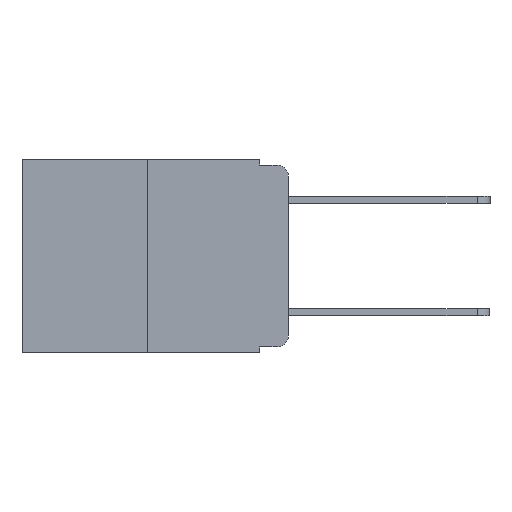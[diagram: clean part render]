
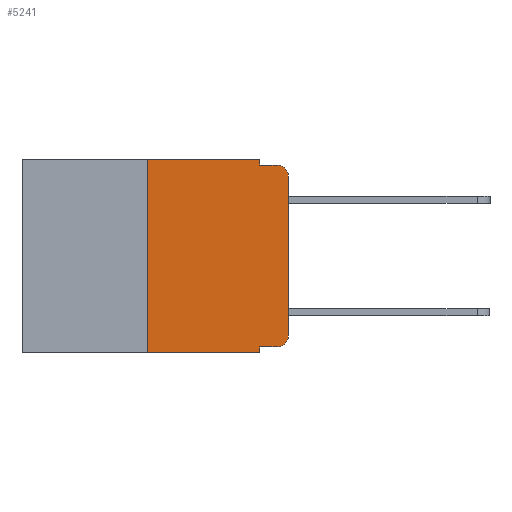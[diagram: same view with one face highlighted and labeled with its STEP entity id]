
A CAD part, left-side view. The second image highlights one B-rep face of the part: STEP entity #5241.
In plain terms, the highlighted planar face has unit normal (-1, 0, 0).
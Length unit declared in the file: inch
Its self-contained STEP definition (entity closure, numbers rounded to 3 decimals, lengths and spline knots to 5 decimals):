
#157 = ORIENTED_EDGE ( 'NONE', *, *, #12236, .F. ) ;
#330 = EDGE_CURVE ( 'NONE', #16093, #11026, #552, .T. ) ;
#552 = LINE ( 'NONE', #17860, #9803 ) ;
#827 = AXIS2_PLACEMENT_3D ( 'NONE', #8892, #20573, #10691 ) ;
#1043 = VERTEX_POINT ( 'NONE', #3173 ) ;
#1145 = VERTEX_POINT ( 'NONE', #20586 ) ;
#1331 = EDGE_CURVE ( 'NONE', #15714, #16093, #13649, .T. ) ;
#1459 = LINE ( 'NONE', #8725, #14645 ) ;
#1630 = CARTESIAN_POINT ( 'NONE',  ( 0., 0.051, -0.333 ) ) ;
#2028 = VECTOR ( 'NONE', #16194, 39.37008 ) ;
#2191 = LINE ( 'NONE', #5204, #19053 ) ;
#2427 = DIRECTION ( 'NONE',  ( 0., 0., 1. ) ) ;
#3173 = CARTESIAN_POINT ( 'NONE',  ( 0., 0., -0.03 ) ) ;
#3844 = LINE ( 'NONE', #4160, #21431 ) ;
#4160 = CARTESIAN_POINT ( 'NONE',  ( 0., 0.25, 0. ) ) ;
#4267 = FACE_OUTER_BOUND ( 'NONE', #19281, .T. ) ;
#4420 = VERTEX_POINT ( 'NONE', #1630 ) ;
#5001 = LINE ( 'NONE', #18997, #13856 ) ;
#5071 = DIRECTION ( 'NONE',  ( 0., 0., -1. ) ) ;
#5204 = CARTESIAN_POINT ( 'NONE',  ( 0., 0.051, -0.333 ) ) ;
#5241 = ADVANCED_FACE ( 'NONE', ( #4267 ), #18147, .F. ) ;
#6113 = ORIENTED_EDGE ( 'NONE', *, *, #330, .F. ) ;
#7399 = DIRECTION ( 'NONE',  ( 0., -1., 0. ) ) ;
#7529 = ORIENTED_EDGE ( 'NONE', *, *, #20690, .T. ) ;
#7534 = CARTESIAN_POINT ( 'NONE',  ( 0., 0.051, -0.01 ) ) ;
#7612 = DIRECTION ( 'NONE',  ( -1., 0., 0. ) ) ;
#8083 = AXIS2_PLACEMENT_3D ( 'NONE', #16545, #19755, #9755 ) ;
#8124 = CARTESIAN_POINT ( 'NONE',  ( 0., 0.051, 0. ) ) ;
#8725 = CARTESIAN_POINT ( 'NONE',  ( 0., 0.051, 0. ) ) ;
#8892 = CARTESIAN_POINT ( 'NONE',  ( 0., 0.02, -0.03 ) ) ;
#8924 = DIRECTION ( 'NONE',  ( 0., -1., 0. ) ) ;
#9149 = EDGE_CURVE ( 'NONE', #18363, #21343, #10734, .T. ) ;
#9168 = CARTESIAN_POINT ( 'NONE',  ( 0., 0.25, 0. ) ) ;
#9550 = CIRCLE ( 'NONE', #12387, 0.02 ) ;
#9646 = ORIENTED_EDGE ( 'NONE', *, *, #16499, .T. ) ;
#9725 = ORIENTED_EDGE ( 'NONE', *, *, #1331, .F. ) ;
#9755 = DIRECTION ( 'NONE',  ( 0., 0., -1. ) ) ;
#9803 = VECTOR ( 'NONE', #7399, 39.37008 ) ;
#10123 = EDGE_CURVE ( 'NONE', #1043, #11026, #12864, .T. ) ;
#10248 = CARTESIAN_POINT ( 'NONE',  ( 0., 0.02, -0.333 ) ) ;
#10691 = DIRECTION ( 'NONE',  ( 0., 0., -1. ) ) ;
#10734 = LINE ( 'NONE', #14883, #19043 ) ;
#11026 = VERTEX_POINT ( 'NONE', #15997 ) ;
#11034 = ORIENTED_EDGE ( 'NONE', *, *, #11558, .F. ) ;
#11558 = EDGE_CURVE ( 'NONE', #4420, #21343, #1459, .T. ) ;
#11722 = VERTEX_POINT ( 'NONE', #9168 ) ;
#12236 = EDGE_CURVE ( 'NONE', #11722, #15714, #5001, .T. ) ;
#12387 = AXIS2_PLACEMENT_3D ( 'NONE', #17790, #7612, #19386 ) ;
#12864 = CIRCLE ( 'NONE', #827, 0.02 ) ;
#13649 = LINE ( 'NONE', #14175, #22176 ) ;
#13788 = CARTESIAN_POINT ( 'NONE',  ( 0., 0.25, -0.343 ) ) ;
#13856 = VECTOR ( 'NONE', #8924, 39.37008 ) ;
#14175 = CARTESIAN_POINT ( 'NONE',  ( 0., 0.051, 0. ) ) ;
#14541 = CARTESIAN_POINT ( 'NONE',  ( 0., 0., 0. ) ) ;
#14645 = VECTOR ( 'NONE', #18827, 39.37008 ) ;
#14883 = CARTESIAN_POINT ( 'NONE',  ( 0., 0.473, -0.343 ) ) ;
#15157 = VERTEX_POINT ( 'NONE', #10248 ) ;
#15586 = ORIENTED_EDGE ( 'NONE', *, *, #17955, .T. ) ;
#15714 = VERTEX_POINT ( 'NONE', #8124 ) ;
#15997 = CARTESIAN_POINT ( 'NONE',  ( 0., 0.02, -0.01 ) ) ;
#16093 = VERTEX_POINT ( 'NONE', #7534 ) ;
#16161 = LINE ( 'NONE', #14541, #2028 ) ;
#16178 = CARTESIAN_POINT ( 'NONE',  ( 0., 0.051, -0.343 ) ) ;
#16194 = DIRECTION ( 'NONE',  ( 0., 0., 1. ) ) ;
#16499 = EDGE_CURVE ( 'NONE', #4420, #15157, #2191, .T. ) ;
#16545 = CARTESIAN_POINT ( 'NONE',  ( 0., 0.473, 0. ) ) ;
#17790 = CARTESIAN_POINT ( 'NONE',  ( 0., 0.02, -0.313 ) ) ;
#17860 = CARTESIAN_POINT ( 'NONE',  ( 0., 0.051, -0.01 ) ) ;
#17955 = EDGE_CURVE ( 'NONE', #15157, #1145, #9550, .T. ) ;
#18137 = DIRECTION ( 'NONE',  ( 0., -1., 0. ) ) ;
#18147 = PLANE ( 'NONE',  #8083 ) ;
#18363 = VERTEX_POINT ( 'NONE', #13788 ) ;
#18654 = ORIENTED_EDGE ( 'NONE', *, *, #10123, .T. ) ;
#18827 = DIRECTION ( 'NONE',  ( 0., 0., -1. ) ) ;
#18879 = DIRECTION ( 'NONE',  ( 0., -1., 0. ) ) ;
#18934 = ORIENTED_EDGE ( 'NONE', *, *, #9149, .T. ) ;
#18997 = CARTESIAN_POINT ( 'NONE',  ( 0., 0.473, 0. ) ) ;
#19043 = VECTOR ( 'NONE', #18137, 39.37008 ) ;
#19053 = VECTOR ( 'NONE', #18879, 39.37008 ) ;
#19281 = EDGE_LOOP ( 'NONE', ( #7529, #18654, #6113, #9725, #157, #21400, #18934, #11034, #9646, #15586 ) ) ;
#19312 = EDGE_CURVE ( 'NONE', #18363, #11722, #3844, .T. ) ;
#19386 = DIRECTION ( 'NONE',  ( 0., 0., -1. ) ) ;
#19755 = DIRECTION ( 'NONE',  ( 1., 0., 0. ) ) ;
#20573 = DIRECTION ( 'NONE',  ( -1., 0., 0. ) ) ;
#20586 = CARTESIAN_POINT ( 'NONE',  ( 0., 0., -0.313 ) ) ;
#20690 = EDGE_CURVE ( 'NONE', #1145, #1043, #16161, .T. ) ;
#21343 = VERTEX_POINT ( 'NONE', #16178 ) ;
#21400 = ORIENTED_EDGE ( 'NONE', *, *, #19312, .F. ) ;
#21431 = VECTOR ( 'NONE', #2427, 39.37008 ) ;
#22176 = VECTOR ( 'NONE', #5071, 39.37008 ) ;
